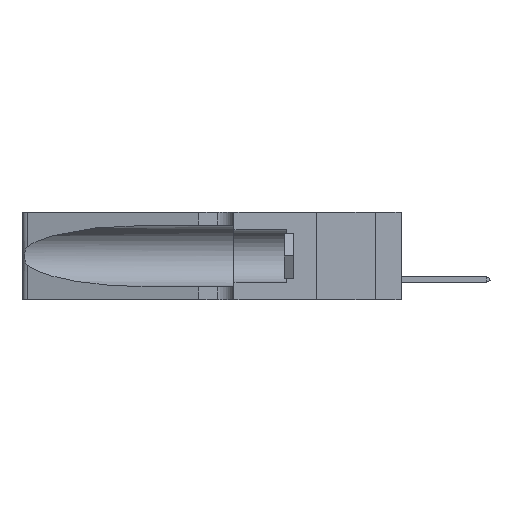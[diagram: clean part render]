
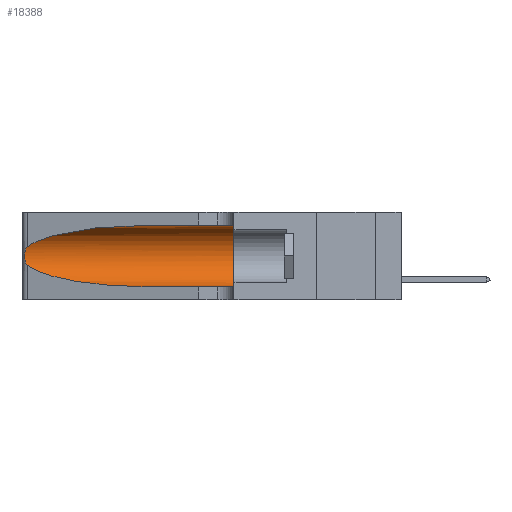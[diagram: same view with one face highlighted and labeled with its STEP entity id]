
A CAD part, left-side view. The second image highlights one B-rep face of the part: STEP entity #18388.
In plain terms, the highlighted cylindrical face has radius 3.308 mm (diameter 6.617 mm), a partial arc.
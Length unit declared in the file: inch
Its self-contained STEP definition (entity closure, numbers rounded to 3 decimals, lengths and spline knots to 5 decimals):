
#667 = EDGE_LOOP ( 'NONE', ( #2494, #40757, #29742, #2280, #38934, #28685 ) ) ;
#2280 = ORIENTED_EDGE ( 'NONE', *, *, #19409, .T. ) ;
#2494 = ORIENTED_EDGE ( 'NONE', *, *, #17517, .T. ) ;
#4009 = CARTESIAN_POINT ( 'NONE',  ( 0.25639, 1.23184, 0.21858 ) ) ;
#4295 = CARTESIAN_POINT ( 'NONE',  ( 0.1305, 1.61858, 0.31525 ) ) ;
#5167 =( BOUNDED_CURVE ( )  B_SPLINE_CURVE ( 3, ( #42205, #46099, #19932, #41081 ),
 .UNSPECIFIED., .F., .T. ) 
 B_SPLINE_CURVE_WITH_KNOTS ( ( 4, 4 ),
 ( 1.5708, 2.84003 ),
 .UNSPECIFIED. ) 
 CURVE ( )  GEOMETRIC_REPRESENTATION_ITEM ( )  RATIONAL_B_SPLINE_CURVE ( ( 1., 0.87, 0.87, 1. ) ) 
 REPRESENTATION_ITEM ( '' )  );
#5830 = CARTESIAN_POINT ( 'NONE',  ( 0.1305, 1.61858, 0.185 ) ) ;
#6429 = VERTEX_POINT ( 'NONE', #35648 ) ;
#6509 = CARTESIAN_POINT ( 'NONE',  ( 0.25487, 1.22718, 0.14631 ) ) ;
#7170 = CARTESIAN_POINT ( 'NONE',  ( 0.2373, 1.15595, 0.08982 ) ) ;
#7564 = CARTESIAN_POINT ( 'NONE',  ( 0.26075, 1.23896, 0.19203 ) ) ;
#7651 = CARTESIAN_POINT ( 'NONE',  ( 0.1305, 0.72297, 0.05475 ) ) ;
#8543 = CYLINDRICAL_SURFACE ( 'NONE', #20295, 0.13025 ) ;
#9158 = DIRECTION ( 'NONE',  ( 0., 0., 1. ) ) ;
#9220 = DIRECTION ( 'NONE',  ( 0., -1., 0. ) ) ;
#9787 = CIRCLE ( 'NONE', #33840, 0.13025 ) ;
#11260 = CARTESIAN_POINT ( 'NONE',  ( 0.25856, 1.23593, 0.16098 ) ) ;
#11751 = CARTESIAN_POINT ( 'NONE',  ( 0.25487, 1.22718, 0.14631 ) ) ;
#11999 = CARTESIAN_POINT ( 'NONE',  ( 0.1305, 1.61858, 0.05475 ) ) ;
#12229 = EDGE_CURVE ( 'NONE', #30250, #23404, #9787, .T. ) ;
#12333 = LINE ( 'NONE', #11999, #25120 ) ;
#15458 = FACE_OUTER_BOUND ( 'NONE', #667, .T. ) ;
#15728 = DIRECTION ( 'NONE',  ( 0., -1., 0. ) ) ;
#16831 = DIRECTION ( 'NONE',  ( 0., 0., -1. ) ) ;
#17517 = EDGE_CURVE ( 'NONE', #28148, #31581, #5167, .T. ) ;
#18388 = ADVANCED_FACE ( 'NONE', ( #15458 ), #8543, .F. ) ;
#18580 = CARTESIAN_POINT ( 'NONE',  ( 0.25787, 1.23484, 0.2124 ) ) ;
#18901 = CARTESIAN_POINT ( 'NONE',  ( 0.25555, 1.22994, 0.2215 ) ) ;
#19054 = CARTESIAN_POINT ( 'NONE',  ( 0.25854, 1.2359, 0.20912 ) ) ;
#19409 = EDGE_CURVE ( 'NONE', #6429, #23404, #12333, .T. ) ;
#19932 = CARTESIAN_POINT ( 'NONE',  ( 0.2373, 1.15595, 0.28018 ) ) ;
#20295 = AXIS2_PLACEMENT_3D ( 'NONE', #5830, #9220, #16831 ) ;
#20966 = B_SPLINE_CURVE_WITH_KNOTS ( 'NONE', 3,
 ( #29834, #18901, #4009, #18580, #19054, #44610, #7564, #44922, #30158, #11260, #30325, #26586, #34057, #11751 ),
 .UNSPECIFIED., .F., .F.,
 ( 4, 2, 2, 2, 2, 2, 4 ),
 ( 0., 0.00027, 0.00053, 0.00107, 0.0016, 0.00187, 0.00214 ),
 .UNSPECIFIED. ) ;
#22275 = CARTESIAN_POINT ( 'NONE',  ( 0.18966, 0.96281, 0.05475 ) ) ;
#23108 = CARTESIAN_POINT ( 'NONE',  ( 0.1305, 0.35, 0.31525 ) ) ;
#23404 = VERTEX_POINT ( 'NONE', #37240 ) ;
#25120 = VECTOR ( 'NONE', #15728, 39.37008 ) ;
#26017 = CARTESIAN_POINT ( 'NONE',  ( 0.25487, 1.22718, 0.14631 ) ) ;
#26586 = CARTESIAN_POINT ( 'NONE',  ( 0.25639, 1.23186, 0.15144 ) ) ;
#27873 = DIRECTION ( 'NONE',  ( 0., 1., 0. ) ) ;
#28148 = VERTEX_POINT ( 'NONE', #43043 ) ;
#28685 = ORIENTED_EDGE ( 'NONE', *, *, #36105, .F. ) ;
#29581 =( BOUNDED_CURVE ( )  B_SPLINE_CURVE ( 3, ( #26017, #7170, #22275, #7651 ),
 .UNSPECIFIED., .F., .T. ) 
 B_SPLINE_CURVE_WITH_KNOTS ( ( 4, 4 ),
 ( 3.44316, 4.71239 ),
 .UNSPECIFIED. ) 
 CURVE ( )  GEOMETRIC_REPRESENTATION_ITEM ( )  RATIONAL_B_SPLINE_CURVE ( ( 1., 0.87, 0.87, 1. ) ) 
 REPRESENTATION_ITEM ( '' )  );
#29742 = ORIENTED_EDGE ( 'NONE', *, *, #30736, .T. ) ;
#29743 = VERTEX_POINT ( 'NONE', #6509 ) ;
#29834 = CARTESIAN_POINT ( 'NONE',  ( 0.25487, 1.22718, 0.22369 ) ) ;
#30158 = CARTESIAN_POINT ( 'NONE',  ( 0.26017, 1.23833, 0.17102 ) ) ;
#30250 = VERTEX_POINT ( 'NONE', #23108 ) ;
#30287 = DIRECTION ( 'NONE',  ( 0., -1., 0. ) ) ;
#30325 = CARTESIAN_POINT ( 'NONE',  ( 0.25789, 1.23486, 0.15765 ) ) ;
#30736 = EDGE_CURVE ( 'NONE', #29743, #6429, #29581, .T. ) ;
#31581 = VERTEX_POINT ( 'NONE', #47364 ) ;
#33167 = VECTOR ( 'NONE', #30287, 39.37008 ) ;
#33840 = AXIS2_PLACEMENT_3D ( 'NONE', #42938, #27873, #9158 ) ;
#34057 = CARTESIAN_POINT ( 'NONE',  ( 0.25555, 1.22993, 0.14849 ) ) ;
#34368 = EDGE_CURVE ( 'NONE', #31581, #29743, #20966, .T. ) ;
#35648 = CARTESIAN_POINT ( 'NONE',  ( 0.1305, 0.72297, 0.05475 ) ) ;
#36105 = EDGE_CURVE ( 'NONE', #28148, #30250, #44220, .T. ) ;
#37240 = CARTESIAN_POINT ( 'NONE',  ( 0.1305, 0.35, 0.05475 ) ) ;
#38934 = ORIENTED_EDGE ( 'NONE', *, *, #12229, .F. ) ;
#40757 = ORIENTED_EDGE ( 'NONE', *, *, #34368, .T. ) ;
#41081 = CARTESIAN_POINT ( 'NONE',  ( 0.25487, 1.22718, 0.22369 ) ) ;
#42205 = CARTESIAN_POINT ( 'NONE',  ( 0.1305, 0.72297, 0.31525 ) ) ;
#42938 = CARTESIAN_POINT ( 'NONE',  ( 0.1305, 0.35, 0.185 ) ) ;
#43043 = CARTESIAN_POINT ( 'NONE',  ( 0.1305, 0.72297, 0.31525 ) ) ;
#44220 = LINE ( 'NONE', #4295, #33167 ) ;
#44610 = CARTESIAN_POINT ( 'NONE',  ( 0.26018, 1.23835, 0.19895 ) ) ;
#44922 = CARTESIAN_POINT ( 'NONE',  ( 0.26075, 1.23896, 0.178 ) ) ;
#46099 = CARTESIAN_POINT ( 'NONE',  ( 0.18966, 0.96281, 0.31525 ) ) ;
#47364 = CARTESIAN_POINT ( 'NONE',  ( 0.25487, 1.22718, 0.22369 ) ) ;
